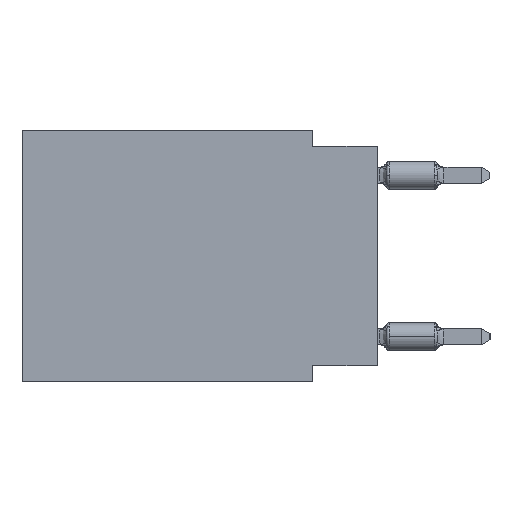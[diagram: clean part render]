
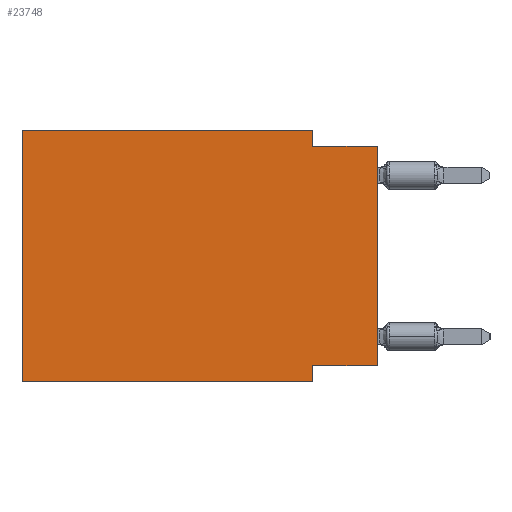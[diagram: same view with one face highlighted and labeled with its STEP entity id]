
A CAD part, left-side view. The second image highlights one B-rep face of the part: STEP entity #23748.
In plain terms, the highlighted planar face has unit normal (-1, 0, 0).
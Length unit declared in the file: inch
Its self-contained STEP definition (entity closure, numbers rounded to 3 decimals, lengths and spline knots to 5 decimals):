
#1441 = DIRECTION ( 'NONE',  ( 0., 0., 1. ) ) ;
#1460 = EDGE_CURVE ( 'NONE', #28094, #11673, #33758, .T. ) ;
#1491 = LINE ( 'NONE', #4258, #2853 ) ;
#1656 = ORIENTED_EDGE ( 'NONE', *, *, #4031, .F. ) ;
#1662 = DIRECTION ( 'NONE',  ( 0., -1., 0. ) ) ;
#2718 = CARTESIAN_POINT ( 'NONE',  ( 0., 0.1, -0.39 ) ) ;
#2810 = EDGE_CURVE ( 'NONE', #7993, #23185, #23809, .T. ) ;
#2853 = VECTOR ( 'NONE', #1662, 39.37008 ) ;
#3009 = VECTOR ( 'NONE', #12356, 39.37008 ) ;
#4031 = EDGE_CURVE ( 'NONE', #11673, #23185, #31598, .T. ) ;
#4258 = CARTESIAN_POINT ( 'NONE',  ( 0., 0.55, 0. ) ) ;
#4563 = CARTESIAN_POINT ( 'NONE',  ( 0., 0.55, -0.39 ) ) ;
#5443 = DIRECTION ( 'NONE',  ( 0., -1., 0. ) ) ;
#5859 = CARTESIAN_POINT ( 'NONE',  ( 0., 0., -0.025 ) ) ;
#6410 = ORIENTED_EDGE ( 'NONE', *, *, #2810, .T. ) ;
#6777 = PLANE ( 'NONE',  #22151 ) ;
#6825 = EDGE_LOOP ( 'NONE', ( #31600, #8661, #30883, #32236, #10176, #6410, #1656, #12842 ) ) ;
#7564 = VECTOR ( 'NONE', #5443, 39.37008 ) ;
#7993 = VERTEX_POINT ( 'NONE', #4563 ) ;
#8024 = CARTESIAN_POINT ( 'NONE',  ( 0., 0., -0.025 ) ) ;
#8661 = ORIENTED_EDGE ( 'NONE', *, *, #29218, .F. ) ;
#9549 = VECTOR ( 'NONE', #10374, 39.37008 ) ;
#10176 = ORIENTED_EDGE ( 'NONE', *, *, #23839, .F. ) ;
#10374 = DIRECTION ( 'NONE',  ( 0., 0., 1. ) ) ;
#10483 = CARTESIAN_POINT ( 'NONE',  ( 0., 0.1, -0.365 ) ) ;
#10755 = CARTESIAN_POINT ( 'NONE',  ( 0., 0.55, -0.39 ) ) ;
#11673 = VERTEX_POINT ( 'NONE', #10483 ) ;
#11916 = FACE_OUTER_BOUND ( 'NONE', #6825, .T. ) ;
#12356 = DIRECTION ( 'NONE',  ( 0., 0., -1. ) ) ;
#12434 = DIRECTION ( 'NONE',  ( 0., 1., 0. ) ) ;
#12842 = ORIENTED_EDGE ( 'NONE', *, *, #1460, .F. ) ;
#13674 = CARTESIAN_POINT ( 'NONE',  ( 0., 0.1, -0.025 ) ) ;
#14647 = DIRECTION ( 'NONE',  ( 1., 0., 0. ) ) ;
#18021 = LINE ( 'NONE', #28858, #3009 ) ;
#18667 = DIRECTION ( 'NONE',  ( 0., 0., -1. ) ) ;
#19503 = CARTESIAN_POINT ( 'NONE',  ( 0., 0.1, -0.39 ) ) ;
#20501 = CARTESIAN_POINT ( 'NONE',  ( 0., 0., -0.365 ) ) ;
#20529 = EDGE_CURVE ( 'NONE', #26946, #31634, #1491, .T. ) ;
#21364 = VECTOR ( 'NONE', #12434, 39.37008 ) ;
#22151 = AXIS2_PLACEMENT_3D ( 'NONE', #30507, #14647, #25152 ) ;
#22201 = CARTESIAN_POINT ( 'NONE',  ( 0., 0., -0.365 ) ) ;
#22264 = VECTOR ( 'NONE', #28292, 39.37008 ) ;
#23185 = VERTEX_POINT ( 'NONE', #19503 ) ;
#23748 = ADVANCED_FACE ( 'NONE', ( #11916 ), #6777, .F. ) ;
#23809 = LINE ( 'NONE', #10755, #22264 ) ;
#23839 = EDGE_CURVE ( 'NONE', #7993, #26946, #28756, .T. ) ;
#24311 = CARTESIAN_POINT ( 'NONE',  ( 0., 0., 0. ) ) ;
#25152 = DIRECTION ( 'NONE',  ( 0., 0., -1. ) ) ;
#25875 = EDGE_CURVE ( 'NONE', #31634, #29163, #18021, .T. ) ;
#26195 = VECTOR ( 'NONE', #1441, 39.37008 ) ;
#26946 = VERTEX_POINT ( 'NONE', #28207 ) ;
#27070 = LINE ( 'NONE', #24311, #26195 ) ;
#28094 = VERTEX_POINT ( 'NONE', #22201 ) ;
#28207 = CARTESIAN_POINT ( 'NONE',  ( 0., 0.55, 0. ) ) ;
#28292 = DIRECTION ( 'NONE',  ( 0., -1., 0. ) ) ;
#28756 = LINE ( 'NONE', #31521, #9549 ) ;
#28858 = CARTESIAN_POINT ( 'NONE',  ( 0., 0.1, 0. ) ) ;
#29163 = VERTEX_POINT ( 'NONE', #13674 ) ;
#29218 = EDGE_CURVE ( 'NONE', #29163, #29963, #31578, .T. ) ;
#29292 = EDGE_CURVE ( 'NONE', #28094, #29963, #27070, .T. ) ;
#29963 = VERTEX_POINT ( 'NONE', #5859 ) ;
#30195 = CARTESIAN_POINT ( 'NONE',  ( 0., 0.1, 0. ) ) ;
#30507 = CARTESIAN_POINT ( 'NONE',  ( 0., 0.55, 0. ) ) ;
#30883 = ORIENTED_EDGE ( 'NONE', *, *, #25875, .F. ) ;
#31521 = CARTESIAN_POINT ( 'NONE',  ( 0., 0.55, 0. ) ) ;
#31578 = LINE ( 'NONE', #8024, #7564 ) ;
#31598 = LINE ( 'NONE', #2718, #32967 ) ;
#31600 = ORIENTED_EDGE ( 'NONE', *, *, #29292, .T. ) ;
#31634 = VERTEX_POINT ( 'NONE', #30195 ) ;
#32236 = ORIENTED_EDGE ( 'NONE', *, *, #20529, .F. ) ;
#32967 = VECTOR ( 'NONE', #18667, 39.37008 ) ;
#33758 = LINE ( 'NONE', #20501, #21364 ) ;
